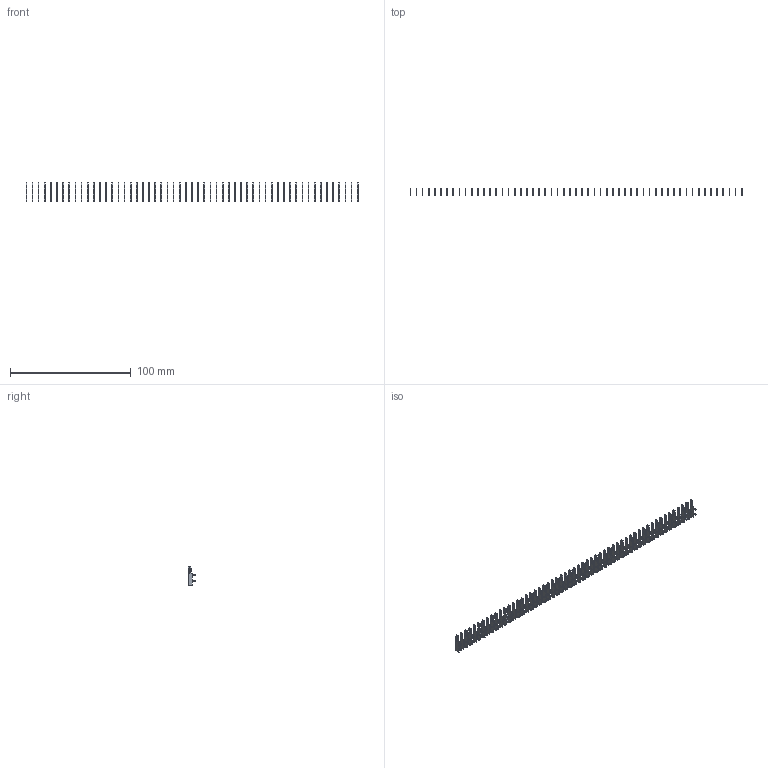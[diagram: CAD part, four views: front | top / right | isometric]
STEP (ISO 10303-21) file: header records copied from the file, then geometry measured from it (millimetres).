
FILE_DESCRIPTION (( 'STEP AP203' ), '1' );
FILE_NAME ('105-055-202-200.STEP', '2020-04-08T00:40:32', ( '' ), ( '' ), 'SwSTEP 2.0', 'SolidWorks 2016', '' );
FILE_SCHEMA (( 'CONFIG_CONTROL_DESIGN' ));
Length unit declared in the file: inch
Products named in the file (2): 100-290-001_100-290-202; 105-055-202-200
Assembly tree (55 placements, depth 2):
  105-055-202-200
    100-290-001_100-290-202  x55
Bounding box: 274.92 x 6.53 x 15.88 mm (x, y, z)
Volume: 1747.5 mm3; surface area: 7771.5 mm2
Topology: 55 solids, 55 shells, 1650 faces, 4620 edges, 3080 vertices
Faces by surface type: plane 1265, cylinder 385
Entity records: 2890 total; most frequent: DIRECTION 270, CARTESIAN_POINT 240, ORIENTED_EDGE 168, CALENDAR_DATE 120, COORDINATED_UNIVERSAL_TIME_OFFSET 120, DATE_AND_TIME 120, LOCAL_TIME 120, AXIS2_PLACEMENT_3D 102
